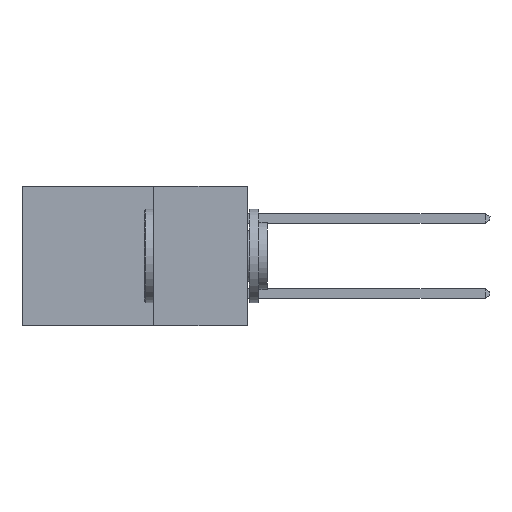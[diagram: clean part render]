
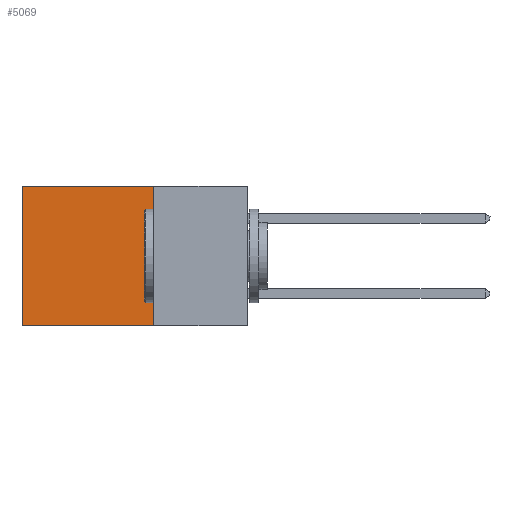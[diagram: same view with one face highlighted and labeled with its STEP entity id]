
A CAD part, left-side view. The second image highlights one B-rep face of the part: STEP entity #5069.
In plain terms, the highlighted planar face has unit normal (-1, 0, 0).
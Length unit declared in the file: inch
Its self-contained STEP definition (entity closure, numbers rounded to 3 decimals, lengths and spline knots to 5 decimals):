
#33 = VERTEX_POINT ( 'NONE', #7236 ) ;
#257 = DIRECTION ( 'NONE',  ( 1., 0., 0. ) ) ;
#427 = VECTOR ( 'NONE', #5824, 39.37008 ) ;
#875 = EDGE_CURVE ( 'NONE', #2861, #33, #6469, .T. ) ;
#1010 = AXIS2_PLACEMENT_3D ( 'NONE', #9204, #257, #3052 ) ;
#1136 = FACE_OUTER_BOUND ( 'NONE', #7935, .T. ) ;
#1251 = EDGE_CURVE ( 'NONE', #8959, #5875, #10721, .T. ) ;
#1365 = ORIENTED_EDGE ( 'NONE', *, *, #875, .T. ) ;
#2681 = ORIENTED_EDGE ( 'NONE', *, *, #5125, .F. ) ;
#2861 = VERTEX_POINT ( 'NONE', #11447 ) ;
#2864 = CARTESIAN_POINT ( 'NONE',  ( 0.2615, 0.25, -0.37 ) ) ;
#3052 = DIRECTION ( 'NONE',  ( 0., 0., -1. ) ) ;
#3345 = EDGE_CURVE ( 'NONE', #33, #5875, #4106, .T. ) ;
#3910 = LINE ( 'NONE', #2864, #5984 ) ;
#4106 = LINE ( 'NONE', #5761, #427 ) ;
#4533 = CARTESIAN_POINT ( 'NONE',  ( 0.2615, 0.6, -0.37 ) ) ;
#4808 = PLANE ( 'NONE',  #1010 ) ;
#4853 = CARTESIAN_POINT ( 'NONE',  ( 0.2615, 0.25, 0. ) ) ;
#5069 = ADVANCED_FACE ( 'NONE', ( #1136 ), #4808, .F. ) ;
#5125 = EDGE_CURVE ( 'NONE', #2861, #8959, #3910, .T. ) ;
#5351 = VECTOR ( 'NONE', #10318, 39.37008 ) ;
#5761 = CARTESIAN_POINT ( 'NONE',  ( 0.2615, 0.6, -0.37 ) ) ;
#5824 = DIRECTION ( 'NONE',  ( 0., 0., -1. ) ) ;
#5875 = VERTEX_POINT ( 'NONE', #4533 ) ;
#5984 = VECTOR ( 'NONE', #6660, 39.37008 ) ;
#6469 = LINE ( 'NONE', #4853, #5351 ) ;
#6660 = DIRECTION ( 'NONE',  ( 0., 0., -1. ) ) ;
#7236 = CARTESIAN_POINT ( 'NONE',  ( 0.2615, 0.6, 0. ) ) ;
#7935 = EDGE_LOOP ( 'NONE', ( #11086, #9218, #2681, #1365 ) ) ;
#8959 = VERTEX_POINT ( 'NONE', #11729 ) ;
#9204 = CARTESIAN_POINT ( 'NONE',  ( 0.2615, 0.25, -0.37 ) ) ;
#9218 = ORIENTED_EDGE ( 'NONE', *, *, #1251, .F. ) ;
#9732 = CARTESIAN_POINT ( 'NONE',  ( 0.2615, 0.25, -0.37 ) ) ;
#10318 = DIRECTION ( 'NONE',  ( 0., 1., 0. ) ) ;
#10666 = DIRECTION ( 'NONE',  ( 0., 1., 0. ) ) ;
#10721 = LINE ( 'NONE', #9732, #10808 ) ;
#10808 = VECTOR ( 'NONE', #10666, 39.37008 ) ;
#11086 = ORIENTED_EDGE ( 'NONE', *, *, #3345, .T. ) ;
#11447 = CARTESIAN_POINT ( 'NONE',  ( 0.2615, 0.25, 0. ) ) ;
#11729 = CARTESIAN_POINT ( 'NONE',  ( 0.2615, 0.25, -0.37 ) ) ;
